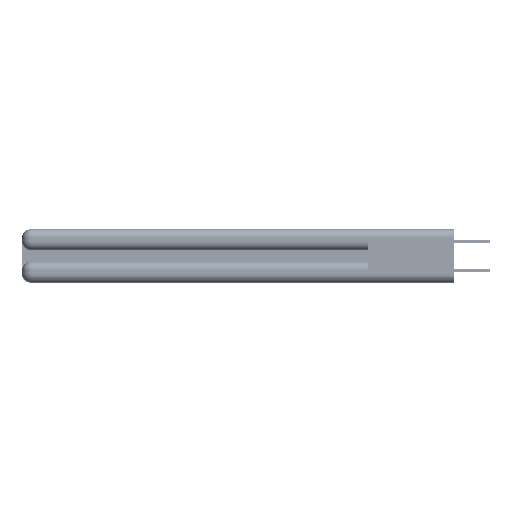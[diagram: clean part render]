
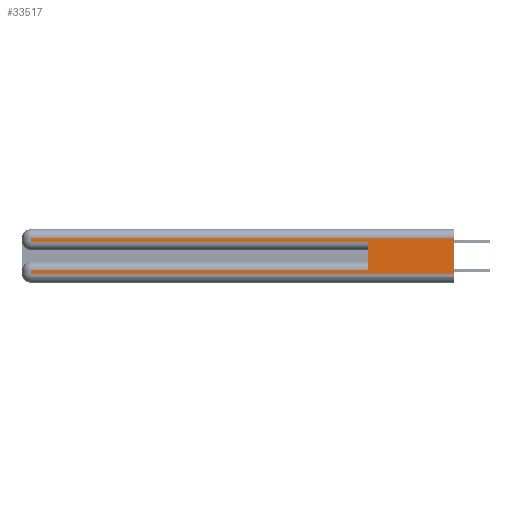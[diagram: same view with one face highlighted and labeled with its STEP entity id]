
A CAD part, left-side view. The second image highlights one B-rep face of the part: STEP entity #33517.
In plain terms, the highlighted planar face has unit normal (-1, 0, 0).
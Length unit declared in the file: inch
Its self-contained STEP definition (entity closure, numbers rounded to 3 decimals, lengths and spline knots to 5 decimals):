
#750 = DIRECTION ( 'NONE',  ( 1., 0., 0. ) ) ;
#2181 = CARTESIAN_POINT ( 'NONE',  ( 0., 2.94, 0.06 ) ) ;
#4550 = CARTESIAN_POINT ( 'NONE',  ( 0., 0., 0.085 ) ) ;
#4656 = EDGE_CURVE ( 'NONE', #23128, #16994, #27414, .T. ) ;
#4979 = VERTEX_POINT ( 'NONE', #27875 ) ;
#5042 = VERTEX_POINT ( 'NONE', #6177 ) ;
#5712 = CARTESIAN_POINT ( 'NONE',  ( 0., 2.94, 0.37 ) ) ;
#6177 = CARTESIAN_POINT ( 'NONE',  ( 0., 0., 0.31 ) ) ;
#6788 = ORIENTED_EDGE ( 'NONE', *, *, #35325, .T. ) ;
#8818 = ORIENTED_EDGE ( 'NONE', *, *, #25168, .T. ) ;
#9320 = DIRECTION ( 'NONE',  ( 0., 0., -1. ) ) ;
#9669 = PLANE ( 'NONE',  #24364 ) ;
#11737 = CARTESIAN_POINT ( 'NONE',  ( 0., 2.94, 0.085 ) ) ;
#14303 = CARTESIAN_POINT ( 'NONE',  ( 0., 0., 0.37 ) ) ;
#14432 = ORIENTED_EDGE ( 'NONE', *, *, #36426, .F. ) ;
#15109 = VECTOR ( 'NONE', #30103, 39.37008 ) ;
#15149 = VECTOR ( 'NONE', #23245, 39.37008 ) ;
#15254 = CARTESIAN_POINT ( 'NONE',  ( 0., 0.6, 0.145 ) ) ;
#15662 = DIRECTION ( 'NONE',  ( 0., 0., -1. ) ) ;
#16994 = VERTEX_POINT ( 'NONE', #2181 ) ;
#17021 = CARTESIAN_POINT ( 'NONE',  ( 0., 0., 0.285 ) ) ;
#17218 = VECTOR ( 'NONE', #25373, 39.37008 ) ;
#19048 = DIRECTION ( 'NONE',  ( 0., 0., -1. ) ) ;
#20178 = EDGE_CURVE ( 'NONE', #40567, #4979, #46951, .T. ) ;
#20252 = CARTESIAN_POINT ( 'NONE',  ( 0., 2.94, 0.285 ) ) ;
#20618 = CARTESIAN_POINT ( 'NONE',  ( 0., 0., 0.31 ) ) ;
#21255 = VERTEX_POINT ( 'NONE', #44678 ) ;
#23128 = VERTEX_POINT ( 'NONE', #11737 ) ;
#23245 = DIRECTION ( 'NONE',  ( 0., 0., 1. ) ) ;
#24364 = AXIS2_PLACEMENT_3D ( 'NONE', #14303, #750, #9320 ) ;
#24557 = LINE ( 'NONE', #4550, #17218 ) ;
#24777 = VECTOR ( 'NONE', #15662, 39.37008 ) ;
#24913 = CARTESIAN_POINT ( 'NONE',  ( 0., 0., 0.06 ) ) ;
#25107 = DIRECTION ( 'NONE',  ( 0., 1., 0. ) ) ;
#25168 = EDGE_CURVE ( 'NONE', #21255, #48610, #43219, .T. ) ;
#25373 = DIRECTION ( 'NONE',  ( 0., 1., 0. ) ) ;
#27414 = LINE ( 'NONE', #41123, #24777 ) ;
#27611 = DIRECTION ( 'NONE',  ( 0., 0., -1. ) ) ;
#27875 = CARTESIAN_POINT ( 'NONE',  ( 0., 0.6, 0.285 ) ) ;
#28267 = ORIENTED_EDGE ( 'NONE', *, *, #50641, .T. ) ;
#29491 = DIRECTION ( 'NONE',  ( 0., -1., 0. ) ) ;
#29508 = EDGE_LOOP ( 'NONE', ( #14432, #6788, #8818, #34068, #50994, #48950, #49547, #28267 ) ) ;
#29734 = CARTESIAN_POINT ( 'NONE',  ( 0., 0., 0.06 ) ) ;
#30103 = DIRECTION ( 'NONE',  ( 0., -1., 0. ) ) ;
#33517 = ADVANCED_FACE ( 'NONE', ( #48720 ), #9669, .F. ) ;
#34068 = ORIENTED_EDGE ( 'NONE', *, *, #40940, .T. ) ;
#35252 = VECTOR ( 'NONE', #27611, 39.37008 ) ;
#35325 = EDGE_CURVE ( 'NONE', #5042, #21255, #38033, .T. ) ;
#36426 = EDGE_CURVE ( 'NONE', #5042, #43813, #51145, .T. ) ;
#36747 = EDGE_CURVE ( 'NONE', #40567, #23128, #24557, .T. ) ;
#38033 = LINE ( 'NONE', #20618, #45326 ) ;
#40301 = CARTESIAN_POINT ( 'NONE',  ( 0., 0.6, 0.085 ) ) ;
#40567 = VERTEX_POINT ( 'NONE', #40301 ) ;
#40627 = CARTESIAN_POINT ( 'NONE',  ( 0., 0., 0.37 ) ) ;
#40940 = EDGE_CURVE ( 'NONE', #48610, #4979, #50175, .T. ) ;
#41123 = CARTESIAN_POINT ( 'NONE',  ( 0., 2.94, 0.37 ) ) ;
#42347 = LINE ( 'NONE', #29734, #15109 ) ;
#43219 = LINE ( 'NONE', #5712, #51800 ) ;
#43813 = VERTEX_POINT ( 'NONE', #24913 ) ;
#44678 = CARTESIAN_POINT ( 'NONE',  ( 0., 2.94, 0.31 ) ) ;
#45326 = VECTOR ( 'NONE', #25107, 39.37008 ) ;
#46951 = LINE ( 'NONE', #15254, #15149 ) ;
#48610 = VERTEX_POINT ( 'NONE', #20252 ) ;
#48720 = FACE_OUTER_BOUND ( 'NONE', #29508, .T. ) ;
#48950 = ORIENTED_EDGE ( 'NONE', *, *, #36747, .T. ) ;
#49487 = VECTOR ( 'NONE', #29491, 39.37008 ) ;
#49547 = ORIENTED_EDGE ( 'NONE', *, *, #4656, .T. ) ;
#50175 = LINE ( 'NONE', #17021, #49487 ) ;
#50641 = EDGE_CURVE ( 'NONE', #16994, #43813, #42347, .T. ) ;
#50994 = ORIENTED_EDGE ( 'NONE', *, *, #20178, .F. ) ;
#51145 = LINE ( 'NONE', #40627, #35252 ) ;
#51800 = VECTOR ( 'NONE', #19048, 39.37008 ) ;
